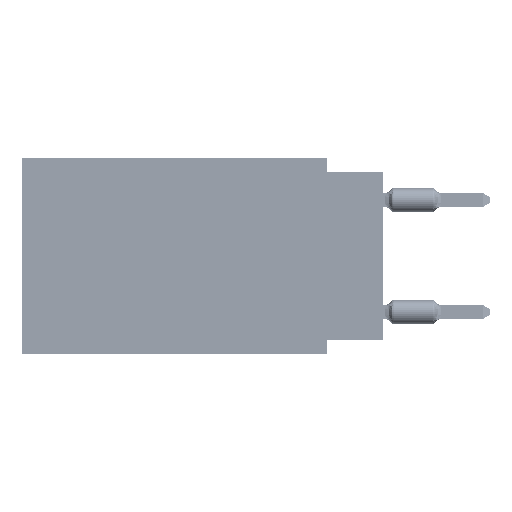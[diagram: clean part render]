
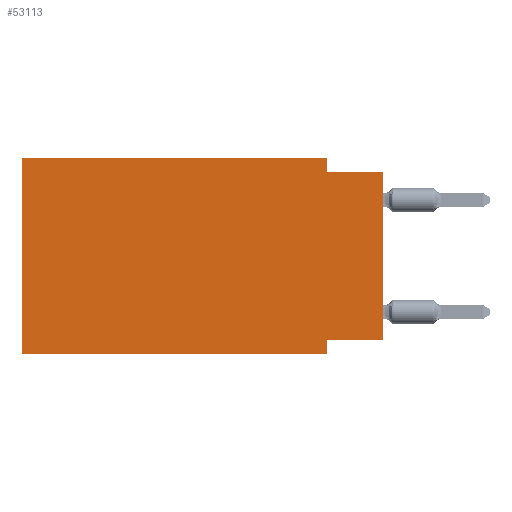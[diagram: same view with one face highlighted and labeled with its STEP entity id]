
A CAD part, left-side view. The second image highlights one B-rep face of the part: STEP entity #53113.
In plain terms, the highlighted planar face has unit normal (-1, 0, 0).
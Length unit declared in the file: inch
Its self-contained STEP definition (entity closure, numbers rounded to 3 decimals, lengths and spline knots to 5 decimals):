
#264 = CARTESIAN_POINT ( 'NONE',  ( 0., 0.1, 0. ) ) ;
#1172 = ORIENTED_EDGE ( 'NONE', *, *, #5742, .F. ) ;
#3585 = LINE ( 'NONE', #84245, #83242 ) ;
#4005 = DIRECTION ( 'NONE',  ( 0., 0., -1. ) ) ;
#5231 = ORIENTED_EDGE ( 'NONE', *, *, #34101, .T. ) ;
#5492 = CARTESIAN_POINT ( 'NONE',  ( 0., 0.1, -0.325 ) ) ;
#5742 = EDGE_CURVE ( 'NONE', #31260, #12440, #102437, .T. ) ;
#6233 = DIRECTION ( 'NONE',  ( 0., -1., 0. ) ) ;
#6316 = LINE ( 'NONE', #75324, #19119 ) ;
#11182 = VERTEX_POINT ( 'NONE', #48295 ) ;
#12440 = VERTEX_POINT ( 'NONE', #93285 ) ;
#14495 = LINE ( 'NONE', #112742, #105231 ) ;
#15593 = VERTEX_POINT ( 'NONE', #28107 ) ;
#19119 = VECTOR ( 'NONE', #4005, 39.37008 ) ;
#21789 = DIRECTION ( 'NONE',  ( 0., 0., 1. ) ) ;
#24558 = CARTESIAN_POINT ( 'NONE',  ( 0., 0., 0. ) ) ;
#26063 = ORIENTED_EDGE ( 'NONE', *, *, #74039, .F. ) ;
#28107 = CARTESIAN_POINT ( 'NONE',  ( 0., 0., -0.325 ) ) ;
#30372 = EDGE_CURVE ( 'NONE', #98570, #11182, #60606, .T. ) ;
#31260 = VERTEX_POINT ( 'NONE', #62498 ) ;
#31608 = VECTOR ( 'NONE', #6233, 39.37008 ) ;
#32373 = CARTESIAN_POINT ( 'NONE',  ( 0., 0.1, -0.025 ) ) ;
#34100 = DIRECTION ( 'NONE',  ( 1., 0., 0. ) ) ;
#34101 = EDGE_CURVE ( 'NONE', #31260, #115357, #78702, .T. ) ;
#37460 = VECTOR ( 'NONE', #21789, 39.37008 ) ;
#39955 = AXIS2_PLACEMENT_3D ( 'NONE', #69768, #34100, #60423 ) ;
#40654 = VECTOR ( 'NONE', #96793, 39.37008 ) ;
#46699 = EDGE_LOOP ( 'NONE', ( #112644, #85007, #84658, #89367, #1172, #5231, #85512, #26063 ) ) ;
#48295 = CARTESIAN_POINT ( 'NONE',  ( 0., 0., -0.025 ) ) ;
#50093 = VERTEX_POINT ( 'NONE', #5492 ) ;
#50766 = DIRECTION ( 'NONE',  ( 0., 1., 0. ) ) ;
#52402 = CARTESIAN_POINT ( 'NONE',  ( 0., 0., -0.025 ) ) ;
#53113 = ADVANCED_FACE ( 'NONE', ( #114213 ), #106565, .F. ) ;
#54634 = CARTESIAN_POINT ( 'NONE',  ( 0., 0.1, -0.35 ) ) ;
#56943 = EDGE_CURVE ( 'NONE', #108058, #98570, #114277, .T. ) ;
#57935 = DIRECTION ( 'NONE',  ( 0., -1., 0. ) ) ;
#59992 = CARTESIAN_POINT ( 'NONE',  ( 0., 0.1, 0. ) ) ;
#60423 = DIRECTION ( 'NONE',  ( 0., 0., -1. ) ) ;
#60606 = LINE ( 'NONE', #52402, #40654 ) ;
#62498 = CARTESIAN_POINT ( 'NONE',  ( 0., 0.645, -0.35 ) ) ;
#68421 = DIRECTION ( 'NONE',  ( 0., 0., 1. ) ) ;
#69637 = VECTOR ( 'NONE', #68421, 39.37008 ) ;
#69768 = CARTESIAN_POINT ( 'NONE',  ( 0., 0.645, 0. ) ) ;
#74039 = EDGE_CURVE ( 'NONE', #15593, #50093, #14495, .T. ) ;
#75324 = CARTESIAN_POINT ( 'NONE',  ( 0., 0.1, -0.35 ) ) ;
#75730 = VECTOR ( 'NONE', #96681, 39.37008 ) ;
#78702 = LINE ( 'NONE', #87454, #31608 ) ;
#83242 = VECTOR ( 'NONE', #57935, 39.37008 ) ;
#84245 = CARTESIAN_POINT ( 'NONE',  ( 0., 0.645, 0. ) ) ;
#84658 = ORIENTED_EDGE ( 'NONE', *, *, #56943, .F. ) ;
#85007 = ORIENTED_EDGE ( 'NONE', *, *, #30372, .F. ) ;
#85512 = ORIENTED_EDGE ( 'NONE', *, *, #85845, .F. ) ;
#85845 = EDGE_CURVE ( 'NONE', #50093, #115357, #6316, .T. ) ;
#87454 = CARTESIAN_POINT ( 'NONE',  ( 0., 0.645, -0.35 ) ) ;
#89367 = ORIENTED_EDGE ( 'NONE', *, *, #109244, .F. ) ;
#93285 = CARTESIAN_POINT ( 'NONE',  ( 0., 0.645, 0. ) ) ;
#95274 = LINE ( 'NONE', #24558, #69637 ) ;
#96681 = DIRECTION ( 'NONE',  ( 0., 0., -1. ) ) ;
#96793 = DIRECTION ( 'NONE',  ( 0., -1., 0. ) ) ;
#98570 = VERTEX_POINT ( 'NONE', #32373 ) ;
#102437 = LINE ( 'NONE', #103618, #37460 ) ;
#103518 = EDGE_CURVE ( 'NONE', #15593, #11182, #95274, .T. ) ;
#103618 = CARTESIAN_POINT ( 'NONE',  ( 0., 0.645, 0. ) ) ;
#105231 = VECTOR ( 'NONE', #50766, 39.37008 ) ;
#106565 = PLANE ( 'NONE',  #39955 ) ;
#108058 = VERTEX_POINT ( 'NONE', #59992 ) ;
#109244 = EDGE_CURVE ( 'NONE', #12440, #108058, #3585, .T. ) ;
#112644 = ORIENTED_EDGE ( 'NONE', *, *, #103518, .T. ) ;
#112742 = CARTESIAN_POINT ( 'NONE',  ( 0., 0., -0.325 ) ) ;
#114213 = FACE_OUTER_BOUND ( 'NONE', #46699, .T. ) ;
#114277 = LINE ( 'NONE', #264, #75730 ) ;
#115357 = VERTEX_POINT ( 'NONE', #54634 ) ;
